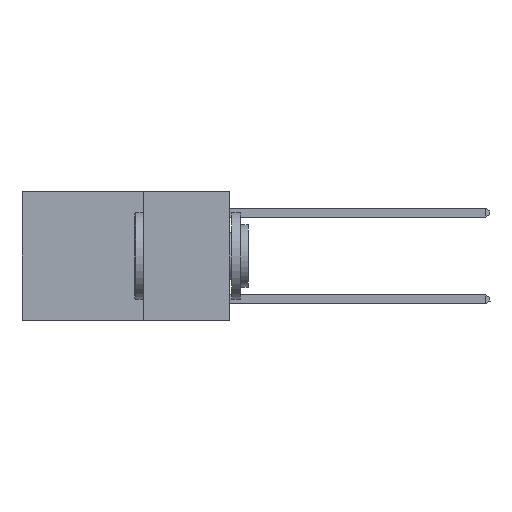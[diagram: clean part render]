
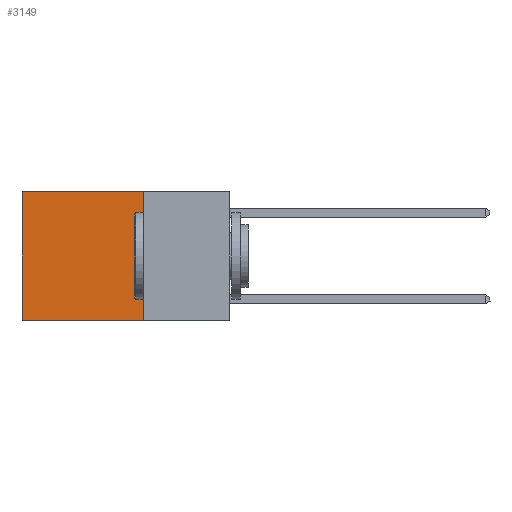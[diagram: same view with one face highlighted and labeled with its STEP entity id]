
A CAD part, left-side view. The second image highlights one B-rep face of the part: STEP entity #3149.
In plain terms, the highlighted planar face has unit normal (-1, 0, 0).
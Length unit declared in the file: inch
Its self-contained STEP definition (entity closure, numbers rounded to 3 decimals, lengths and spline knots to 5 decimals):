
#163 = VECTOR ( 'NONE', #11483, 39.37008 ) ;
#259 = AXIS2_PLACEMENT_3D ( 'NONE', #3281, #6560, #5049 ) ;
#1814 = DIRECTION ( 'NONE',  ( 0., 1., 0. ) ) ;
#2104 = LINE ( 'NONE', #5146, #7941 ) ;
#2148 = VERTEX_POINT ( 'NONE', #12200 ) ;
#2899 = EDGE_CURVE ( 'NONE', #2148, #7324, #11166, .T. ) ;
#3149 = ADVANCED_FACE ( 'NONE', ( #13141 ), #13092, .F. ) ;
#3281 = CARTESIAN_POINT ( 'NONE',  ( 0.2625, 0.25, 0. ) ) ;
#3461 = LINE ( 'NONE', #4928, #163 ) ;
#3576 = LINE ( 'NONE', #9676, #9053 ) ;
#4218 = DIRECTION ( 'NONE',  ( 0., 1., 0. ) ) ;
#4704 = CARTESIAN_POINT ( 'NONE',  ( 0.2625, 0.25, 0. ) ) ;
#4928 = CARTESIAN_POINT ( 'NONE',  ( 0.2625, 0.6, 0. ) ) ;
#5049 = DIRECTION ( 'NONE',  ( 0., 0., -1. ) ) ;
#5146 = CARTESIAN_POINT ( 'NONE',  ( 0.2625, 0.25, 0. ) ) ;
#6560 = DIRECTION ( 'NONE',  ( 1., 0., 0. ) ) ;
#6734 = EDGE_CURVE ( 'NONE', #12940, #7324, #3461, .T. ) ;
#7220 = CARTESIAN_POINT ( 'NONE',  ( 0.2625, 0.25, -0.37 ) ) ;
#7324 = VERTEX_POINT ( 'NONE', #8017 ) ;
#7647 = EDGE_LOOP ( 'NONE', ( #13518, #13618, #13660, #13686 ) ) ;
#7889 = VECTOR ( 'NONE', #1814, 39.37008 ) ;
#7941 = VECTOR ( 'NONE', #12780, 39.37008 ) ;
#8017 = CARTESIAN_POINT ( 'NONE',  ( 0.2625, 0.6, -0.37 ) ) ;
#8904 = EDGE_CURVE ( 'NONE', #10443, #12940, #3576, .T. ) ;
#9053 = VECTOR ( 'NONE', #4218, 39.37008 ) ;
#9676 = CARTESIAN_POINT ( 'NONE',  ( 0.2625, 0.25, 0. ) ) ;
#10443 = VERTEX_POINT ( 'NONE', #4704 ) ;
#11166 = LINE ( 'NONE', #7220, #7889 ) ;
#11483 = DIRECTION ( 'NONE',  ( 0., 0., -1. ) ) ;
#12200 = CARTESIAN_POINT ( 'NONE',  ( 0.2625, 0.25, -0.37 ) ) ;
#12780 = DIRECTION ( 'NONE',  ( 0., 0., -1. ) ) ;
#12940 = VERTEX_POINT ( 'NONE', #13401 ) ;
#13092 = PLANE ( 'NONE',  #259 ) ;
#13141 = FACE_OUTER_BOUND ( 'NONE', #7647, .T. ) ;
#13401 = CARTESIAN_POINT ( 'NONE',  ( 0.2625, 0.6, 0. ) ) ;
#13518 = ORIENTED_EDGE ( 'NONE', *, *, #6734, .T. ) ;
#13618 = ORIENTED_EDGE ( 'NONE', *, *, #2899, .F. ) ;
#13660 = ORIENTED_EDGE ( 'NONE', *, *, #14111, .F. ) ;
#13686 = ORIENTED_EDGE ( 'NONE', *, *, #8904, .T. ) ;
#14111 = EDGE_CURVE ( 'NONE', #10443, #2148, #2104, .T. ) ;
